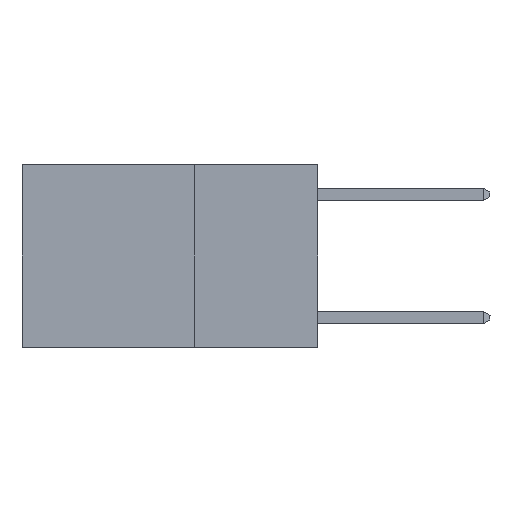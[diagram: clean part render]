
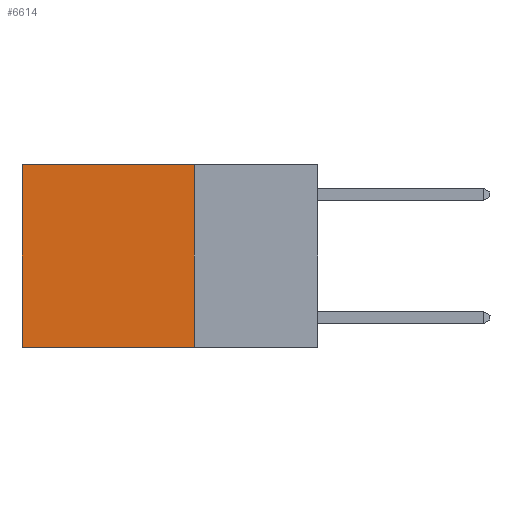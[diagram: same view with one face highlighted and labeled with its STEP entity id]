
A CAD part, left-side view. The second image highlights one B-rep face of the part: STEP entity #6614.
In plain terms, the highlighted planar face has unit normal (-1, 0, 0).
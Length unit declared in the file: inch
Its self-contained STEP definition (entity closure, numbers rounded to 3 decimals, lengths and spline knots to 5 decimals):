
#3 = CARTESIAN_POINT ( 'NONE',  ( 0.2625, 0.25, 0. ) ) ;
#15 = CARTESIAN_POINT ( 'NONE',  ( 0.2625, 0.6, 0. ) ) ;
#101 = DIRECTION ( 'NONE',  ( 0., 0., -1. ) ) ;
#141 = LINE ( 'NONE', #1296, #5690 ) ;
#219 = DIRECTION ( 'NONE',  ( 0., 0., -1. ) ) ;
#355 = VECTOR ( 'NONE', #4874, 39.37008 ) ;
#716 = CARTESIAN_POINT ( 'NONE',  ( 0.2625, 0.25, 0. ) ) ;
#947 = CARTESIAN_POINT ( 'NONE',  ( 0.2625, 0.6, -0.37 ) ) ;
#1135 = EDGE_LOOP ( 'NONE', ( #3486, #8512, #5399, #6686 ) ) ;
#1296 = CARTESIAN_POINT ( 'NONE',  ( 0.2625, 0.25, 0. ) ) ;
#1358 = FACE_OUTER_BOUND ( 'NONE', #1135, .T. ) ;
#1761 = EDGE_CURVE ( 'NONE', #2635, #3724, #7475, .T. ) ;
#2635 = VERTEX_POINT ( 'NONE', #7649 ) ;
#3202 = LINE ( 'NONE', #15, #355 ) ;
#3476 = LINE ( 'NONE', #716, #9078 ) ;
#3486 = ORIENTED_EDGE ( 'NONE', *, *, #6206, .T. ) ;
#3718 = PLANE ( 'NONE',  #7312 ) ;
#3724 = VERTEX_POINT ( 'NONE', #947 ) ;
#3817 = CARTESIAN_POINT ( 'NONE',  ( 0.2625, 0.25, 0. ) ) ;
#4601 = CARTESIAN_POINT ( 'NONE',  ( 0.2625, 0.25, -0.37 ) ) ;
#4874 = DIRECTION ( 'NONE',  ( 0., 0., -1. ) ) ;
#4886 = EDGE_CURVE ( 'NONE', #8691, #2635, #3476, .T. ) ;
#5399 = ORIENTED_EDGE ( 'NONE', *, *, #4886, .F. ) ;
#5690 = VECTOR ( 'NONE', #6941, 39.37008 ) ;
#5791 = CARTESIAN_POINT ( 'NONE',  ( 0.2625, 0.6, 0. ) ) ;
#6206 = EDGE_CURVE ( 'NONE', #9044, #3724, #3202, .T. ) ;
#6614 = ADVANCED_FACE ( 'NONE', ( #1358 ), #3718, .F. ) ;
#6686 = ORIENTED_EDGE ( 'NONE', *, *, #8547, .T. ) ;
#6941 = DIRECTION ( 'NONE',  ( 0., 1., 0. ) ) ;
#7312 = AXIS2_PLACEMENT_3D ( 'NONE', #3817, #8747, #219 ) ;
#7475 = LINE ( 'NONE', #4601, #8721 ) ;
#7649 = CARTESIAN_POINT ( 'NONE',  ( 0.2625, 0.25, -0.37 ) ) ;
#8204 = DIRECTION ( 'NONE',  ( 0., 1., 0. ) ) ;
#8512 = ORIENTED_EDGE ( 'NONE', *, *, #1761, .F. ) ;
#8547 = EDGE_CURVE ( 'NONE', #8691, #9044, #141, .T. ) ;
#8691 = VERTEX_POINT ( 'NONE', #3 ) ;
#8721 = VECTOR ( 'NONE', #8204, 39.37008 ) ;
#8747 = DIRECTION ( 'NONE',  ( 1., 0., 0. ) ) ;
#9044 = VERTEX_POINT ( 'NONE', #5791 ) ;
#9078 = VECTOR ( 'NONE', #101, 39.37008 ) ;
